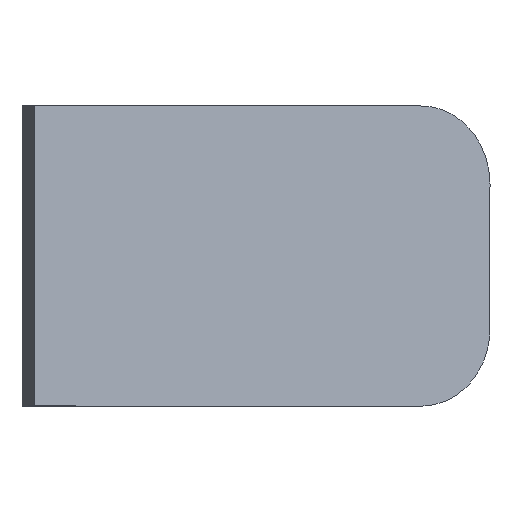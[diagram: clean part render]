
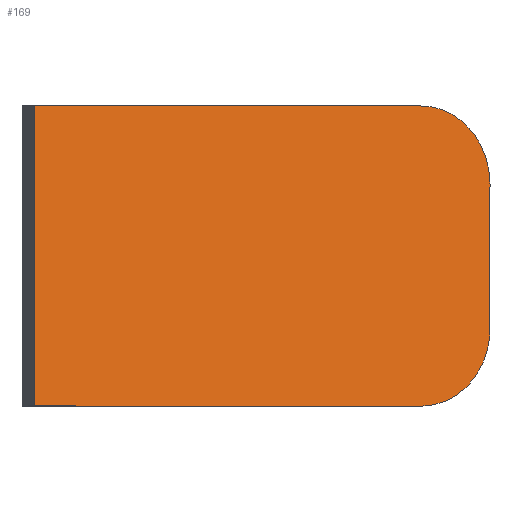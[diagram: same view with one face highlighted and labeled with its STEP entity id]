
A CAD part, top view. The second image highlights one B-rep face of the part: STEP entity #169.
In plain terms, the highlighted planar face has unit normal (0.376, 0, 0.927).
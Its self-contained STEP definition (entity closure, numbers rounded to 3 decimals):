
#17=B_SPLINE_CURVE_WITH_KNOTS('',3,(#304,#305,#306,#307,#308,#309,#310,
#311,#312,#313,#314,#315,#316,#317,#318,#319),.UNSPECIFIED.,.F.,.F.,(4,
3,3,3,3,4),(-0.783,-0.681,-0.573,-0.379,
-0.187,0.),.UNSPECIFIED.);
#19=B_SPLINE_CURVE_WITH_KNOTS('',3,(#368,#369,#370,#371,#372,#373,#374,
#375,#376,#377,#378,#379,#380),.UNSPECIFIED.,.F.,.F.,(4,3,3,3,4),(-0.785,
-0.599,-0.409,-0.208,0.),
 .UNSPECIFIED.);
#28=PLANE('',#193);
#38=FACE_OUTER_BOUND('',#49,.T.);
#49=EDGE_LOOP('',(#153,#154,#155,#156,#157,#158));
#53=LINE('',#246,#68);
#56=LINE('',#252,#71);
#60=LINE('',#325,#75);
#64=LINE('',#384,#79);
#68=VECTOR('',#209,10.);
#71=VECTOR('',#214,10.);
#75=VECTOR('',#220,10.);
#79=VECTOR('',#226,10.);
#86=VERTEX_POINT('',#243);
#87=VERTEX_POINT('',#245);
#89=VERTEX_POINT('',#251);
#91=VERTEX_POINT('',#303);
#93=VERTEX_POINT('',#324);
#95=VERTEX_POINT('',#367);
#101=EDGE_CURVE('',#87,#86,#53,.T.);
#104=EDGE_CURVE('',#89,#87,#56,.T.);
#107=EDGE_CURVE('',#91,#89,#17,.T.);
#110=EDGE_CURVE('',#93,#91,#60,.T.);
#113=EDGE_CURVE('',#95,#93,#19,.T.);
#116=EDGE_CURVE('',#86,#95,#64,.T.);
#153=ORIENTED_EDGE('',*,*,#116,.T.);
#154=ORIENTED_EDGE('',*,*,#113,.T.);
#155=ORIENTED_EDGE('',*,*,#110,.T.);
#156=ORIENTED_EDGE('',*,*,#107,.T.);
#157=ORIENTED_EDGE('',*,*,#104,.T.);
#158=ORIENTED_EDGE('',*,*,#101,.T.);
#169=ADVANCED_FACE('',(#38),#28,.F.);
#193=AXIS2_PLACEMENT_3D('',#386,#229,#230);
#209=DIRECTION('',(0.,-1.,0.));
#214=DIRECTION('',(-0.927,0.,0.376));
#220=DIRECTION('',(0.,1.,0.));
#226=DIRECTION('',(0.927,0.,-0.376));
#229=DIRECTION('center_axis',(-0.376,0.,
-0.927));
#230=DIRECTION('ref_axis',(0.,-1.,0.));
#243=CARTESIAN_POINT('',(49.67,13.622,19.275));
#245=CARTESIAN_POINT('',(49.67,31.599,19.275));
#246=CARTESIAN_POINT('',(49.67,31.853,19.275));
#251=CARTESIAN_POINT('',(72.791,31.599,9.899));
#252=CARTESIAN_POINT('',(72.791,31.599,9.899));
#303=CARTESIAN_POINT('',(76.938,26.924,8.217));
#304=CARTESIAN_POINT('Ctrl Pts',(76.938,26.924,8.217));
#305=CARTESIAN_POINT('Ctrl Pts',(76.938,27.239,8.217));
#306=CARTESIAN_POINT('Ctrl Pts',(76.91,27.554,8.228));
#307=CARTESIAN_POINT('Ctrl Pts',(76.854,27.863,8.251));
#308=CARTESIAN_POINT('Ctrl Pts',(76.794,28.191,8.275));
#309=CARTESIAN_POINT('Ctrl Pts',(76.703,28.511,8.312));
#310=CARTESIAN_POINT('Ctrl Pts',(76.582,28.819,8.361));
#311=CARTESIAN_POINT('Ctrl Pts',(76.367,29.367,8.449));
#312=CARTESIAN_POINT('Ctrl Pts',(76.059,29.866,8.574));
#313=CARTESIAN_POINT('Ctrl Pts',(75.672,30.287,8.73));
#314=CARTESIAN_POINT('Ctrl Pts',(75.287,30.706,8.886));
#315=CARTESIAN_POINT('Ctrl Pts',(74.831,31.04,9.071));
#316=CARTESIAN_POINT('Ctrl Pts',(74.329,31.266,9.275));
#317=CARTESIAN_POINT('Ctrl Pts',(73.84,31.486,9.473));
#318=CARTESIAN_POINT('Ctrl Pts',(73.319,31.599,9.684));
#319=CARTESIAN_POINT('Ctrl Pts',(72.791,31.599,9.899));
#324=CARTESIAN_POINT('',(76.938,18.297,8.217));
#325=CARTESIAN_POINT('',(76.938,18.297,8.217));
#367=CARTESIAN_POINT('',(72.791,13.622,9.899));
#368=CARTESIAN_POINT('Ctrl Pts',(72.791,13.622,9.899));
#369=CARTESIAN_POINT('Ctrl Pts',(73.314,13.622,9.687));
#370=CARTESIAN_POINT('Ctrl Pts',(73.83,13.733,9.477));
#371=CARTESIAN_POINT('Ctrl Pts',(74.314,13.948,9.281));
#372=CARTESIAN_POINT('Ctrl Pts',(74.81,14.169,9.08));
#373=CARTESIAN_POINT('Ctrl Pts',(75.261,14.495,8.897));
#374=CARTESIAN_POINT('Ctrl Pts',(75.644,14.904,8.742));
#375=CARTESIAN_POINT('Ctrl Pts',(76.051,15.339,8.577));
#376=CARTESIAN_POINT('Ctrl Pts',(76.373,15.859,8.446));
#377=CARTESIAN_POINT('Ctrl Pts',(76.594,16.432,8.356));
#378=CARTESIAN_POINT('Ctrl Pts',(76.821,17.022,8.264));
#379=CARTESIAN_POINT('Ctrl Pts',(76.938,17.657,8.217));
#380=CARTESIAN_POINT('Ctrl Pts',(76.938,18.297,8.217));
#384=CARTESIAN_POINT('',(72.791,13.622,9.899));
#386=CARTESIAN_POINT('Origin',(63.304,22.61,13.746));
